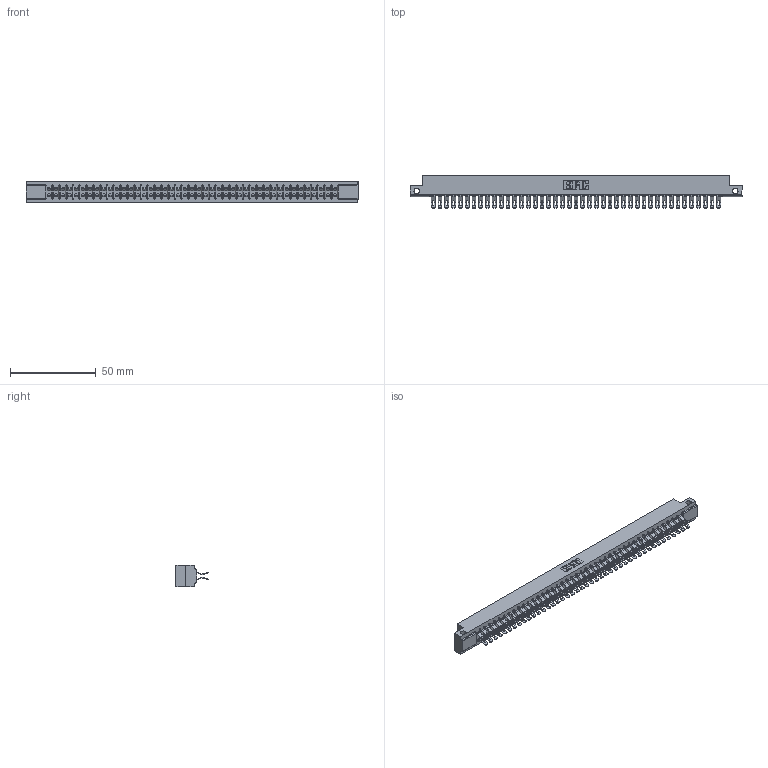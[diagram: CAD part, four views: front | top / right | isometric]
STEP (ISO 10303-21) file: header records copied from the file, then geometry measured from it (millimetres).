
FILE_DESCRIPTION (( 'STEP AP203' ), '1' );
FILE_NAME ('357-086-555-212.STEP', '2018-08-13T02:39:30', ( '' ), ( '' ), 'SwSTEP 2.0', 'SolidWorks 2016', '' );
FILE_SCHEMA (( 'CONFIG_CONTROL_DESIGN' ));
Length unit declared in the file: inch
Products named in the file (3): 307 Part_.128 Dia Side Mounting Holes; 307-290-001_555; 357-086-555-212
Assembly tree (87 placements, depth 2):
  357-086-555-212
    307 Part_.128 Dia Side Mounting Holes
    307-290-001_555  x86
Bounding box: 193.4 x 18.75 x 12.7 mm (x, y, z)
Volume: 20686.5 mm3; surface area: 26739 mm2
Topology: 87 solids, 87 shells, 5408 faces, 15889 edges, 10358 vertices
Faces by surface type: plane 2994, cylinder 2326, sphere 88
Entity records: 38655 total; most frequent: CARTESIAN_POINT 6327, ORIENTED_EDGE 6272, DIRECTION 6204, EDGE_CURVE 3136, LINE 2394, VECTOR 2394, VERTEX_POINT 2028, AXIS2_PLACEMENT_3D 1905
